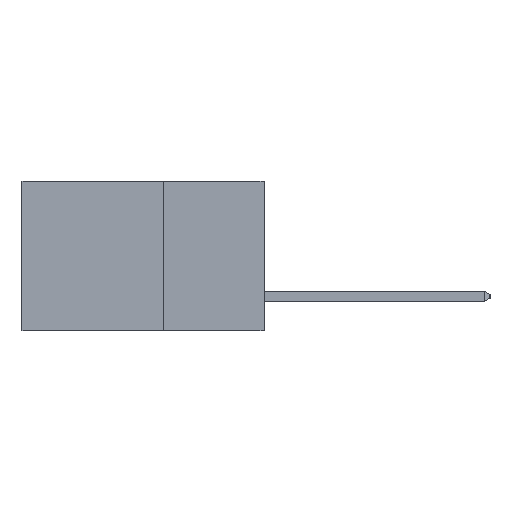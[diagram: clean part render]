
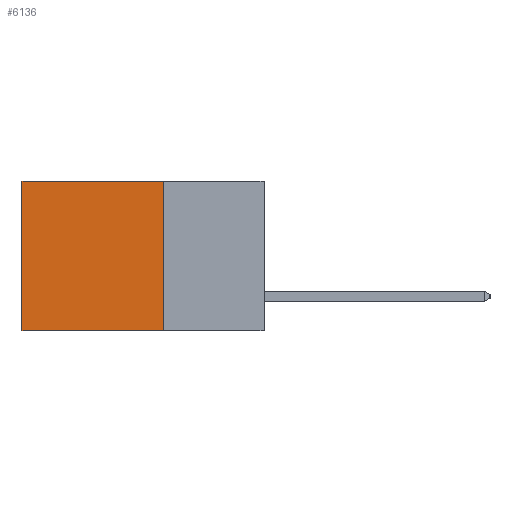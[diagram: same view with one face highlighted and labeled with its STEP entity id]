
A CAD part, left-side view. The second image highlights one B-rep face of the part: STEP entity #6136.
In plain terms, the highlighted planar face has unit normal (-1, 0, 0).
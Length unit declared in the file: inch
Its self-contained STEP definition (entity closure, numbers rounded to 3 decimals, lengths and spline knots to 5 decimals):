
#363 = VECTOR ( 'NONE', #7140, 39.37008 ) ;
#831 = ORIENTED_EDGE ( 'NONE', *, *, #8976, .F. ) ;
#900 = ORIENTED_EDGE ( 'NONE', *, *, #10431, .F. ) ;
#1189 = EDGE_CURVE ( 'NONE', #2756, #12468, #9507, .T. ) ;
#2415 = CARTESIAN_POINT ( 'NONE',  ( 0.298, 0.25, 0. ) ) ;
#2756 = VERTEX_POINT ( 'NONE', #10975 ) ;
#3390 = CARTESIAN_POINT ( 'NONE',  ( 0.298, 0.25, 0. ) ) ;
#4821 = CARTESIAN_POINT ( 'NONE',  ( 0.298, 0.25, 0. ) ) ;
#4859 = EDGE_CURVE ( 'NONE', #12267, #2756, #6280, .T. ) ;
#5513 = FACE_OUTER_BOUND ( 'NONE', #9047, .T. ) ;
#5864 = CARTESIAN_POINT ( 'NONE',  ( 0.298, 0.25, -0.37 ) ) ;
#6130 = LINE ( 'NONE', #3390, #12045 ) ;
#6136 = ADVANCED_FACE ( 'NONE', ( #5513 ), #14236, .F. ) ;
#6242 = ORIENTED_EDGE ( 'NONE', *, *, #1189, .T. ) ;
#6280 = LINE ( 'NONE', #4821, #9442 ) ;
#7140 = DIRECTION ( 'NONE',  ( 0., 0., -1. ) ) ;
#7300 = CARTESIAN_POINT ( 'NONE',  ( 0.298, 0.6, 0. ) ) ;
#7302 = DIRECTION ( 'NONE',  ( 0., 1., 0. ) ) ;
#7446 = VECTOR ( 'NONE', #7302, 39.37008 ) ;
#7479 = AXIS2_PLACEMENT_3D ( 'NONE', #14248, #14309, #14294 ) ;
#7490 = CARTESIAN_POINT ( 'NONE',  ( 0.298, 0.6, -0.37 ) ) ;
#7555 = ORIENTED_EDGE ( 'NONE', *, *, #4859, .T. ) ;
#7827 = LINE ( 'NONE', #12009, #7446 ) ;
#8976 = EDGE_CURVE ( 'NONE', #13620, #12468, #7827, .T. ) ;
#9047 = EDGE_LOOP ( 'NONE', ( #6242, #831, #900, #7555 ) ) ;
#9442 = VECTOR ( 'NONE', #14855, 39.37008 ) ;
#9507 = LINE ( 'NONE', #7300, #363 ) ;
#10431 = EDGE_CURVE ( 'NONE', #12267, #13620, #6130, .T. ) ;
#10520 = DIRECTION ( 'NONE',  ( 0., 0., -1. ) ) ;
#10975 = CARTESIAN_POINT ( 'NONE',  ( 0.298, 0.6, 0. ) ) ;
#12009 = CARTESIAN_POINT ( 'NONE',  ( 0.298, 0.25, -0.37 ) ) ;
#12045 = VECTOR ( 'NONE', #10520, 39.37008 ) ;
#12267 = VERTEX_POINT ( 'NONE', #2415 ) ;
#12468 = VERTEX_POINT ( 'NONE', #7490 ) ;
#13620 = VERTEX_POINT ( 'NONE', #5864 ) ;
#14236 = PLANE ( 'NONE',  #7479 ) ;
#14248 = CARTESIAN_POINT ( 'NONE',  ( 0.298, 0.25, 0. ) ) ;
#14294 = DIRECTION ( 'NONE',  ( 0., 0., -1. ) ) ;
#14309 = DIRECTION ( 'NONE',  ( 1., 0., 0. ) ) ;
#14855 = DIRECTION ( 'NONE',  ( 0., 1., 0. ) ) ;
